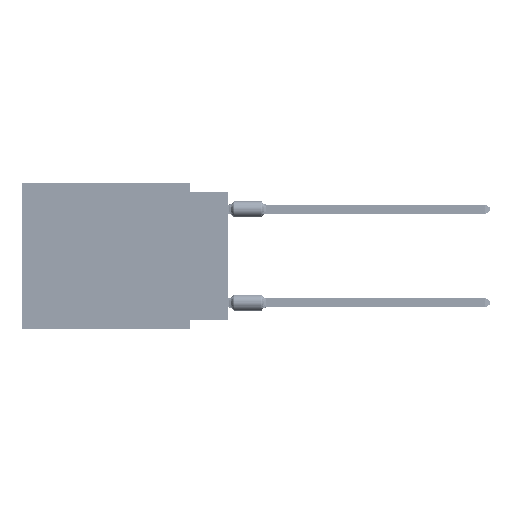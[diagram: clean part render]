
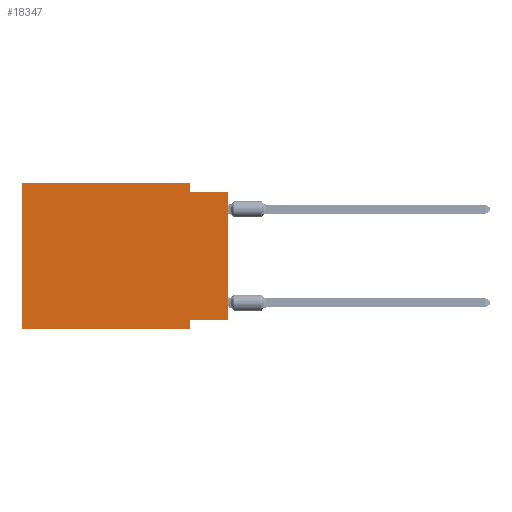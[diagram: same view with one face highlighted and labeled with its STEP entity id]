
A CAD part, left-side view. The second image highlights one B-rep face of the part: STEP entity #18347.
In plain terms, the highlighted planar face has unit normal (-1, 0, 0).
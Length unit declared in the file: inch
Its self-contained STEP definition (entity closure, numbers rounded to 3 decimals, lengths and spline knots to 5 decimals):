
#1035 = EDGE_CURVE ( 'NONE', #61891, #3742, #29692, .T. ) ;
#1138 = LINE ( 'NONE', #17857, #42088 ) ;
#1154 = CARTESIAN_POINT ( 'NONE',  ( 0., 0.1, 0. ) ) ;
#2008 = CARTESIAN_POINT ( 'NONE',  ( 0., 0.1, -0.025 ) ) ;
#2484 = DIRECTION ( 'NONE',  ( 0., -1., 0. ) ) ;
#3742 = VERTEX_POINT ( 'NONE', #23670 ) ;
#7399 = VECTOR ( 'NONE', #29118, 39.37008 ) ;
#10319 = EDGE_CURVE ( 'NONE', #63613, #36038, #1138, .T. ) ;
#10445 = CARTESIAN_POINT ( 'NONE',  ( 0., 0.1, -0.39 ) ) ;
#12267 = CARTESIAN_POINT ( 'NONE',  ( 0., 0., 0. ) ) ;
#12585 = CARTESIAN_POINT ( 'NONE',  ( 0., 0.55, -0.39 ) ) ;
#14634 = EDGE_CURVE ( 'NONE', #63613, #43793, #25224, .T. ) ;
#14985 = LINE ( 'NONE', #10445, #56329 ) ;
#15004 = CARTESIAN_POINT ( 'NONE',  ( 0., 0., -0.365 ) ) ;
#16352 = EDGE_LOOP ( 'NONE', ( #35567, #64799, #42969, #34839, #68728, #68874, #42278, #23045 ) ) ;
#17857 = CARTESIAN_POINT ( 'NONE',  ( 0., 0.55, -0.39 ) ) ;
#18048 = CARTESIAN_POINT ( 'NONE',  ( 0., 0.1, -0.365 ) ) ;
#18347 = ADVANCED_FACE ( 'NONE', ( #65785 ), #49399, .F. ) ;
#18453 = EDGE_CURVE ( 'NONE', #64183, #36038, #14985, .T. ) ;
#18509 = CARTESIAN_POINT ( 'NONE',  ( 0., 0., -0.025 ) ) ;
#18594 = DIRECTION ( 'NONE',  ( 0., 0., -1. ) ) ;
#20167 = EDGE_CURVE ( 'NONE', #39620, #64183, #41588, .T. ) ;
#20267 = VECTOR ( 'NONE', #33565, 39.37008 ) ;
#22434 = DIRECTION ( 'NONE',  ( 0., 0., -1. ) ) ;
#23045 = ORIENTED_EDGE ( 'NONE', *, *, #20167, .F. ) ;
#23288 = DIRECTION ( 'NONE',  ( 0., -1., 0. ) ) ;
#23670 = CARTESIAN_POINT ( 'NONE',  ( 0., 0., -0.025 ) ) ;
#23839 = CARTESIAN_POINT ( 'NONE',  ( 0., 0.55, 0. ) ) ;
#25224 = LINE ( 'NONE', #66492, #7399 ) ;
#27845 = CARTESIAN_POINT ( 'NONE',  ( 0., 0.55, 0. ) ) ;
#29118 = DIRECTION ( 'NONE',  ( 0., 0., 1. ) ) ;
#29692 = LINE ( 'NONE', #18509, #58575 ) ;
#30518 = CARTESIAN_POINT ( 'NONE',  ( 0., 0.1, 0. ) ) ;
#31747 = DIRECTION ( 'NONE',  ( 0., 0., -1. ) ) ;
#32916 = DIRECTION ( 'NONE',  ( 0., -1., 0. ) ) ;
#33565 = DIRECTION ( 'NONE',  ( 0., 0., 1. ) ) ;
#34142 = LINE ( 'NONE', #27845, #53818 ) ;
#34839 = ORIENTED_EDGE ( 'NONE', *, *, #55931, .F. ) ;
#35567 = ORIENTED_EDGE ( 'NONE', *, *, #53426, .T. ) ;
#36038 = VERTEX_POINT ( 'NONE', #67603 ) ;
#39077 = CARTESIAN_POINT ( 'NONE',  ( 0., 0.55, 0. ) ) ;
#39620 = VERTEX_POINT ( 'NONE', #48459 ) ;
#41588 = LINE ( 'NONE', #15004, #65406 ) ;
#42088 = VECTOR ( 'NONE', #32916, 39.37008 ) ;
#42278 = ORIENTED_EDGE ( 'NONE', *, *, #18453, .F. ) ;
#42969 = ORIENTED_EDGE ( 'NONE', *, *, #60121, .F. ) ;
#43793 = VERTEX_POINT ( 'NONE', #39077 ) ;
#44324 = VECTOR ( 'NONE', #22434, 39.37008 ) ;
#45189 = DIRECTION ( 'NONE',  ( 1., 0., 0. ) ) ;
#48459 = CARTESIAN_POINT ( 'NONE',  ( 0., 0., -0.365 ) ) ;
#49014 = LINE ( 'NONE', #1154, #44324 ) ;
#49399 = PLANE ( 'NONE',  #55250 ) ;
#49638 = LINE ( 'NONE', #12267, #20267 ) ;
#53426 = EDGE_CURVE ( 'NONE', #39620, #3742, #49638, .T. ) ;
#53818 = VECTOR ( 'NONE', #23288, 39.37008 ) ;
#55250 = AXIS2_PLACEMENT_3D ( 'NONE', #23839, #45189, #18594 ) ;
#55931 = EDGE_CURVE ( 'NONE', #43793, #59949, #34142, .T. ) ;
#56329 = VECTOR ( 'NONE', #31747, 39.37008 ) ;
#58575 = VECTOR ( 'NONE', #2484, 39.37008 ) ;
#59949 = VERTEX_POINT ( 'NONE', #30518 ) ;
#60121 = EDGE_CURVE ( 'NONE', #59949, #61891, #49014, .T. ) ;
#61891 = VERTEX_POINT ( 'NONE', #2008 ) ;
#63613 = VERTEX_POINT ( 'NONE', #12585 ) ;
#64183 = VERTEX_POINT ( 'NONE', #18048 ) ;
#64799 = ORIENTED_EDGE ( 'NONE', *, *, #1035, .F. ) ;
#65406 = VECTOR ( 'NONE', #68457, 39.37008 ) ;
#65785 = FACE_OUTER_BOUND ( 'NONE', #16352, .T. ) ;
#66492 = CARTESIAN_POINT ( 'NONE',  ( 0., 0.55, 0. ) ) ;
#67603 = CARTESIAN_POINT ( 'NONE',  ( 0., 0.1, -0.39 ) ) ;
#68457 = DIRECTION ( 'NONE',  ( 0., 1., 0. ) ) ;
#68728 = ORIENTED_EDGE ( 'NONE', *, *, #14634, .F. ) ;
#68874 = ORIENTED_EDGE ( 'NONE', *, *, #10319, .T. ) ;
